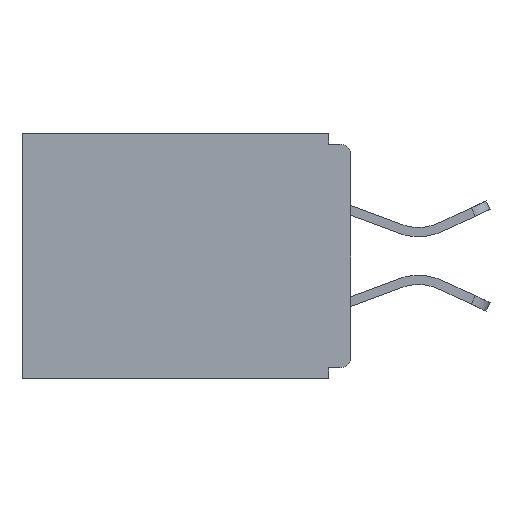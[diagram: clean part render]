
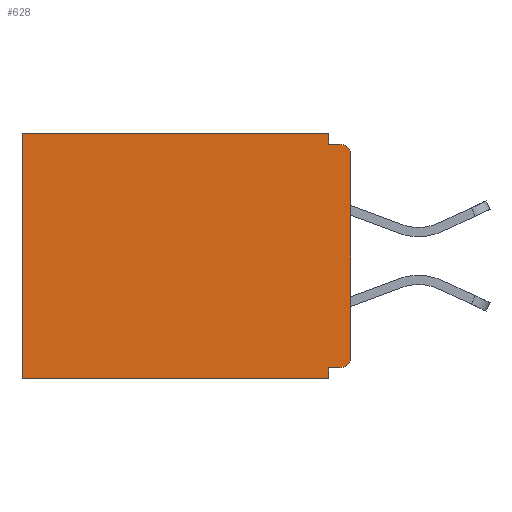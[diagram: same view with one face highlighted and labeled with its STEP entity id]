
A CAD part, left-side view. The second image highlights one B-rep face of the part: STEP entity #628.
In plain terms, the highlighted planar face has unit normal (-1, 0, 0).
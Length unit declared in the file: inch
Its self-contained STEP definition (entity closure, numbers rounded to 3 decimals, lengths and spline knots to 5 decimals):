
#116 = DIRECTION ( 'NONE',  ( 0., 0., -1. ) ) ;
#424 = VERTEX_POINT ( 'NONE', #10410 ) ;
#499 = AXIS2_PLACEMENT_3D ( 'NONE', #23329, #10493, #1780 ) ;
#515 = CARTESIAN_POINT ( 'NONE',  ( 0.298, 0., -0.343 ) ) ;
#566 = ORIENTED_EDGE ( 'NONE', *, *, #12075, .T. ) ;
#628 = ADVANCED_FACE ( 'NONE', ( #13332 ), #21527, .F. ) ;
#851 = CARTESIAN_POINT ( 'NONE',  ( 0.298, 0., -0.328 ) ) ;
#974 = ORIENTED_EDGE ( 'NONE', *, *, #22841, .F. ) ;
#1106 = EDGE_CURVE ( 'NONE', #7001, #21671, #8502, .T. ) ;
#1780 = DIRECTION ( 'NONE',  ( 0., 0., -1. ) ) ;
#1822 = LINE ( 'NONE', #3574, #13932 ) ;
#1892 = DIRECTION ( 'NONE',  ( 0., -1., 0. ) ) ;
#2303 = DIRECTION ( 'NONE',  ( 0., 0., -1. ) ) ;
#2652 = CARTESIAN_POINT ( 'NONE',  ( 0.298, 0.031, -0.343 ) ) ;
#2800 = ORIENTED_EDGE ( 'NONE', *, *, #7176, .T. ) ;
#3082 = ORIENTED_EDGE ( 'NONE', *, *, #3534, .F. ) ;
#3324 = AXIS2_PLACEMENT_3D ( 'NONE', #16177, #16423, #18233 ) ;
#3327 = VECTOR ( 'NONE', #10259, 39.37008 ) ;
#3469 = CARTESIAN_POINT ( 'NONE',  ( 0.298, 0.015, -0.015 ) ) ;
#3534 = EDGE_CURVE ( 'NONE', #8788, #9869, #21595, .T. ) ;
#3574 = CARTESIAN_POINT ( 'NONE',  ( 0.298, 0.46, 0. ) ) ;
#3975 = ORIENTED_EDGE ( 'NONE', *, *, #6264, .F. ) ;
#4091 = ORIENTED_EDGE ( 'NONE', *, *, #16512, .F. ) ;
#4646 = VERTEX_POINT ( 'NONE', #18424 ) ;
#5158 = CARTESIAN_POINT ( 'NONE',  ( 0.298, 0., 0. ) ) ;
#5510 = DIRECTION ( 'NONE',  ( 0., 1., 0. ) ) ;
#5575 = VERTEX_POINT ( 'NONE', #7802 ) ;
#6264 = EDGE_CURVE ( 'NONE', #19104, #424, #10003, .T. ) ;
#6746 = LINE ( 'NONE', #5158, #22511 ) ;
#6813 = ORIENTED_EDGE ( 'NONE', *, *, #23015, .T. ) ;
#7001 = VERTEX_POINT ( 'NONE', #13706 ) ;
#7176 = EDGE_CURVE ( 'NONE', #10859, #424, #1822, .T. ) ;
#7209 = VECTOR ( 'NONE', #5510, 39.37008 ) ;
#7398 = CARTESIAN_POINT ( 'NONE',  ( 0.298, 0., -0.015 ) ) ;
#7680 = CARTESIAN_POINT ( 'NONE',  ( 0.298, 0.031, -0.343 ) ) ;
#7802 = CARTESIAN_POINT ( 'NONE',  ( 0.298, 0.031, -0.015 ) ) ;
#7935 = VECTOR ( 'NONE', #116, 39.37008 ) ;
#8502 = LINE ( 'NONE', #9091, #7935 ) ;
#8514 = CARTESIAN_POINT ( 'NONE',  ( 0.298, 0.46, 0. ) ) ;
#8788 = VERTEX_POINT ( 'NONE', #13851 ) ;
#9091 = CARTESIAN_POINT ( 'NONE',  ( 0.298, 0., 0. ) ) ;
#9245 = ORIENTED_EDGE ( 'NONE', *, *, #19723, .F. ) ;
#9869 = VERTEX_POINT ( 'NONE', #20172 ) ;
#9910 = CIRCLE ( 'NONE', #3324, 0.015 ) ;
#9982 = DIRECTION ( 'NONE',  ( 0., 1., 0. ) ) ;
#10003 = LINE ( 'NONE', #515, #7209 ) ;
#10259 = DIRECTION ( 'NONE',  ( 0., 0., -1. ) ) ;
#10410 = CARTESIAN_POINT ( 'NONE',  ( 0.298, 0.46, -0.343 ) ) ;
#10493 = DIRECTION ( 'NONE',  ( 1., 0., 0. ) ) ;
#10661 = ORIENTED_EDGE ( 'NONE', *, *, #1106, .F. ) ;
#10859 = VERTEX_POINT ( 'NONE', #8514 ) ;
#11889 = VECTOR ( 'NONE', #2303, 39.37008 ) ;
#12075 = EDGE_CURVE ( 'NONE', #4646, #10859, #6746, .T. ) ;
#12148 = CARTESIAN_POINT ( 'NONE',  ( 0.298, 0.031, -0.343 ) ) ;
#12298 = VECTOR ( 'NONE', #9982, 39.37008 ) ;
#12761 = CARTESIAN_POINT ( 'NONE',  ( 0.298, 0.015, -0.03 ) ) ;
#13332 = FACE_OUTER_BOUND ( 'NONE', #20513, .T. ) ;
#13706 = CARTESIAN_POINT ( 'NONE',  ( 0.298, 0., -0.03 ) ) ;
#13851 = CARTESIAN_POINT ( 'NONE',  ( 0.298, 0.015, -0.328 ) ) ;
#13868 = VECTOR ( 'NONE', #1892, 39.37008 ) ;
#13932 = VECTOR ( 'NONE', #17632, 39.37008 ) ;
#14430 = DIRECTION ( 'NONE',  ( -1., 0., 0. ) ) ;
#15316 = LINE ( 'NONE', #7680, #11889 ) ;
#15411 = LINE ( 'NONE', #12148, #3327 ) ;
#16177 = CARTESIAN_POINT ( 'NONE',  ( 0.298, 0.015, -0.313 ) ) ;
#16423 = DIRECTION ( 'NONE',  ( -1., 0., 0. ) ) ;
#16512 = EDGE_CURVE ( 'NONE', #4646, #5575, #15316, .T. ) ;
#16739 = CIRCLE ( 'NONE', #22923, 0.015 ) ;
#17513 = VERTEX_POINT ( 'NONE', #3469 ) ;
#17632 = DIRECTION ( 'NONE',  ( 0., 0., -1. ) ) ;
#17839 = CARTESIAN_POINT ( 'NONE',  ( 0.298, 0., -0.313 ) ) ;
#18233 = DIRECTION ( 'NONE',  ( 0., 0., -1. ) ) ;
#18396 = LINE ( 'NONE', #7398, #13868 ) ;
#18424 = CARTESIAN_POINT ( 'NONE',  ( 0.298, 0.031, 0. ) ) ;
#18711 = ORIENTED_EDGE ( 'NONE', *, *, #22031, .T. ) ;
#19104 = VERTEX_POINT ( 'NONE', #2652 ) ;
#19723 = EDGE_CURVE ( 'NONE', #9869, #19104, #15411, .T. ) ;
#20172 = CARTESIAN_POINT ( 'NONE',  ( 0.298, 0.031, -0.328 ) ) ;
#20513 = EDGE_LOOP ( 'NONE', ( #18711, #974, #4091, #566, #2800, #3975, #9245, #3082, #6813, #10661 ) ) ;
#21253 = DIRECTION ( 'NONE',  ( 0., 1., 0. ) ) ;
#21527 = PLANE ( 'NONE',  #499 ) ;
#21595 = LINE ( 'NONE', #851, #12298 ) ;
#21671 = VERTEX_POINT ( 'NONE', #17839 ) ;
#21896 = DIRECTION ( 'NONE',  ( 0., 0., -1. ) ) ;
#22031 = EDGE_CURVE ( 'NONE', #7001, #17513, #16739, .T. ) ;
#22511 = VECTOR ( 'NONE', #21253, 39.37008 ) ;
#22841 = EDGE_CURVE ( 'NONE', #5575, #17513, #18396, .T. ) ;
#22923 = AXIS2_PLACEMENT_3D ( 'NONE', #12761, #14430, #21896 ) ;
#23015 = EDGE_CURVE ( 'NONE', #8788, #21671, #9910, .T. ) ;
#23329 = CARTESIAN_POINT ( 'NONE',  ( 0.298, 0., 0. ) ) ;
